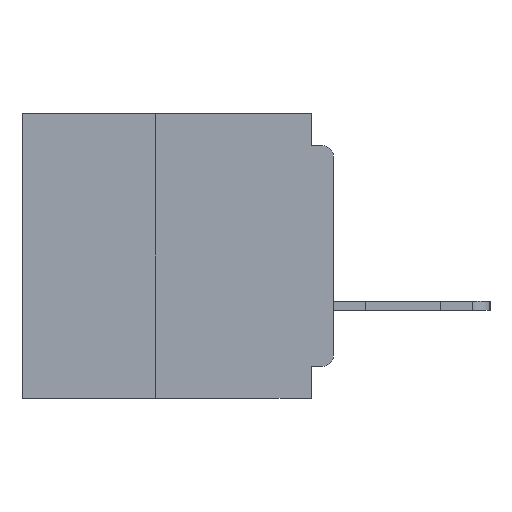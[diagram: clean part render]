
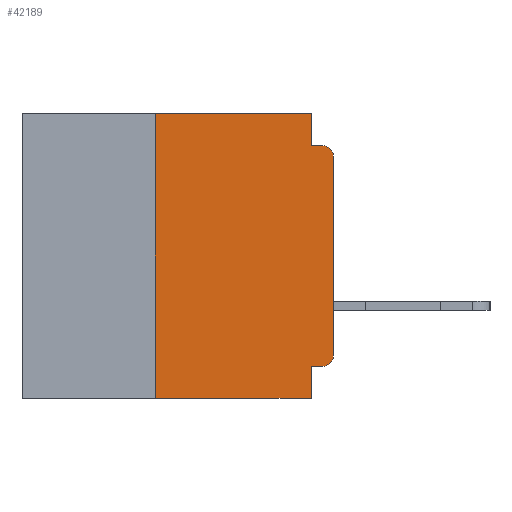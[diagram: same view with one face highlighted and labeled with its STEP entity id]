
A CAD part, left-side view. The second image highlights one B-rep face of the part: STEP entity #42189.
In plain terms, the highlighted planar face has unit normal (-1, 0, 0).
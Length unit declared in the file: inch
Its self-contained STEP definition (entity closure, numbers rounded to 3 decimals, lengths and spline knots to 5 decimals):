
#959 = ORIENTED_EDGE ( 'NONE', *, *, #11011, .F. ) ;
#1242 = EDGE_CURVE ( 'NONE', #25947, #39227, #44777, .T. ) ;
#1860 = ORIENTED_EDGE ( 'NONE', *, *, #31243, .F. ) ;
#2241 = CARTESIAN_POINT ( 'NONE',  ( 0., 0.015, -0.355 ) ) ;
#2334 = DIRECTION ( 'NONE',  ( 0., 0., -1. ) ) ;
#2494 = CARTESIAN_POINT ( 'NONE',  ( 0., 0.437, 0. ) ) ;
#3840 = VERTEX_POINT ( 'NONE', #31394 ) ;
#3915 = LINE ( 'NONE', #25311, #42820 ) ;
#3919 = DIRECTION ( 'NONE',  ( 0., 0., 1. ) ) ;
#4160 = VECTOR ( 'NONE', #8870, 39.37008 ) ;
#5090 = CARTESIAN_POINT ( 'NONE',  ( 0., 0.25, 0. ) ) ;
#5402 = EDGE_CURVE ( 'NONE', #23320, #25947, #29004, .T. ) ;
#6300 = DIRECTION ( 'NONE',  ( 1., 0., 0. ) ) ;
#6639 = CARTESIAN_POINT ( 'NONE',  ( 0., 0.031, -0.045 ) ) ;
#8055 = ORIENTED_EDGE ( 'NONE', *, *, #13537, .T. ) ;
#8590 = LINE ( 'NONE', #28203, #27472 ) ;
#8870 = DIRECTION ( 'NONE',  ( 0., 0., 1. ) ) ;
#10076 = DIRECTION ( 'NONE',  ( 0., -1., 0. ) ) ;
#10105 = VECTOR ( 'NONE', #3919, 39.37008 ) ;
#11011 = EDGE_CURVE ( 'NONE', #45464, #48167, #3915, .T. ) ;
#13124 = CARTESIAN_POINT ( 'NONE',  ( 0., 0., -0.34 ) ) ;
#13537 = EDGE_CURVE ( 'NONE', #3840, #48167, #14823, .T. ) ;
#13640 = VECTOR ( 'NONE', #38287, 39.37008 ) ;
#14066 = DIRECTION ( 'NONE',  ( -1., 0., 0. ) ) ;
#14158 = LINE ( 'NONE', #39010, #4160 ) ;
#14823 = LINE ( 'NONE', #23107, #13640 ) ;
#14967 = VECTOR ( 'NONE', #47777, 39.37008 ) ;
#15282 = CARTESIAN_POINT ( 'NONE',  ( 0., 0., -0.06 ) ) ;
#16404 = EDGE_CURVE ( 'NONE', #31903, #45464, #26186, .T. ) ;
#16922 = EDGE_LOOP ( 'NONE', ( #29794, #30994, #46046, #1860, #42005, #32177, #8055, #959, #23980, #24919 ) ) ;
#17264 = AXIS2_PLACEMENT_3D ( 'NONE', #24054, #14066, #2334 ) ;
#17503 = CARTESIAN_POINT ( 'NONE',  ( 0., 0.015, -0.045 ) ) ;
#17627 = CARTESIAN_POINT ( 'NONE',  ( 0., 0.437, 0. ) ) ;
#18687 = VERTEX_POINT ( 'NONE', #5090 ) ;
#20631 = AXIS2_PLACEMENT_3D ( 'NONE', #2494, #6300, #32656 ) ;
#20731 = VECTOR ( 'NONE', #34517, 39.37008 ) ;
#21264 = VECTOR ( 'NONE', #10076, 39.37008 ) ;
#22450 = DIRECTION ( 'NONE',  ( -1., 0., 0. ) ) ;
#22828 = CARTESIAN_POINT ( 'NONE',  ( 0., 0., 0. ) ) ;
#23107 = CARTESIAN_POINT ( 'NONE',  ( 0., 0.437, -0.4 ) ) ;
#23320 = VERTEX_POINT ( 'NONE', #13124 ) ;
#23845 = AXIS2_PLACEMENT_3D ( 'NONE', #45047, #22450, #48787 ) ;
#23980 = ORIENTED_EDGE ( 'NONE', *, *, #16404, .F. ) ;
#24054 = CARTESIAN_POINT ( 'NONE',  ( 0., 0.015, -0.06 ) ) ;
#24606 = EDGE_CURVE ( 'NONE', #18687, #44060, #41334, .T. ) ;
#24919 = ORIENTED_EDGE ( 'NONE', *, *, #45150, .T. ) ;
#25311 = CARTESIAN_POINT ( 'NONE',  ( 0., 0.031, -0.4 ) ) ;
#25947 = VERTEX_POINT ( 'NONE', #15282 ) ;
#26186 = LINE ( 'NONE', #44183, #14967 ) ;
#27472 = VECTOR ( 'NONE', #43345, 39.37008 ) ;
#28203 = CARTESIAN_POINT ( 'NONE',  ( 0., 0.031, 0. ) ) ;
#28742 = EDGE_CURVE ( 'NONE', #3840, #18687, #14158, .T. ) ;
#29004 = LINE ( 'NONE', #22828, #10105 ) ;
#29794 = ORIENTED_EDGE ( 'NONE', *, *, #5402, .T. ) ;
#30755 = CARTESIAN_POINT ( 'NONE',  ( 0., 0., -0.045 ) ) ;
#30994 = ORIENTED_EDGE ( 'NONE', *, *, #1242, .T. ) ;
#31243 = EDGE_CURVE ( 'NONE', #44060, #45652, #8590, .T. ) ;
#31394 = CARTESIAN_POINT ( 'NONE',  ( 0., 0.25, -0.4 ) ) ;
#31903 = VERTEX_POINT ( 'NONE', #2241 ) ;
#32177 = ORIENTED_EDGE ( 'NONE', *, *, #28742, .F. ) ;
#32656 = DIRECTION ( 'NONE',  ( 0., 0., -1. ) ) ;
#34517 = DIRECTION ( 'NONE',  ( 0., -1., 0. ) ) ;
#36078 = FACE_OUTER_BOUND ( 'NONE', #16922, .T. ) ;
#36527 = DIRECTION ( 'NONE',  ( 0., 0., -1. ) ) ;
#36640 = EDGE_CURVE ( 'NONE', #45652, #39227, #40816, .T. ) ;
#36919 = CARTESIAN_POINT ( 'NONE',  ( 0., 0.031, 0. ) ) ;
#37619 = CIRCLE ( 'NONE', #23845, 0.015 ) ;
#38287 = DIRECTION ( 'NONE',  ( 0., -1., 0. ) ) ;
#39010 = CARTESIAN_POINT ( 'NONE',  ( 0., 0.25, -0.4 ) ) ;
#39227 = VERTEX_POINT ( 'NONE', #17503 ) ;
#39231 = CARTESIAN_POINT ( 'NONE',  ( 0., 0.031, -0.355 ) ) ;
#39533 = CARTESIAN_POINT ( 'NONE',  ( 0., 0.031, -0.4 ) ) ;
#40052 = PLANE ( 'NONE',  #20631 ) ;
#40816 = LINE ( 'NONE', #30755, #20731 ) ;
#41334 = LINE ( 'NONE', #17627, #21264 ) ;
#42005 = ORIENTED_EDGE ( 'NONE', *, *, #24606, .F. ) ;
#42189 = ADVANCED_FACE ( 'NONE', ( #36078 ), #40052, .F. ) ;
#42820 = VECTOR ( 'NONE', #36527, 39.37008 ) ;
#43345 = DIRECTION ( 'NONE',  ( 0., 0., -1. ) ) ;
#44060 = VERTEX_POINT ( 'NONE', #36919 ) ;
#44183 = CARTESIAN_POINT ( 'NONE',  ( 0., 0., -0.355 ) ) ;
#44777 = CIRCLE ( 'NONE', #17264, 0.015 ) ;
#45047 = CARTESIAN_POINT ( 'NONE',  ( 0., 0.015, -0.34 ) ) ;
#45150 = EDGE_CURVE ( 'NONE', #31903, #23320, #37619, .T. ) ;
#45464 = VERTEX_POINT ( 'NONE', #39231 ) ;
#45652 = VERTEX_POINT ( 'NONE', #6639 ) ;
#46046 = ORIENTED_EDGE ( 'NONE', *, *, #36640, .F. ) ;
#47777 = DIRECTION ( 'NONE',  ( 0., 1., 0. ) ) ;
#48167 = VERTEX_POINT ( 'NONE', #39533 ) ;
#48787 = DIRECTION ( 'NONE',  ( 0., 0., -1. ) ) ;
